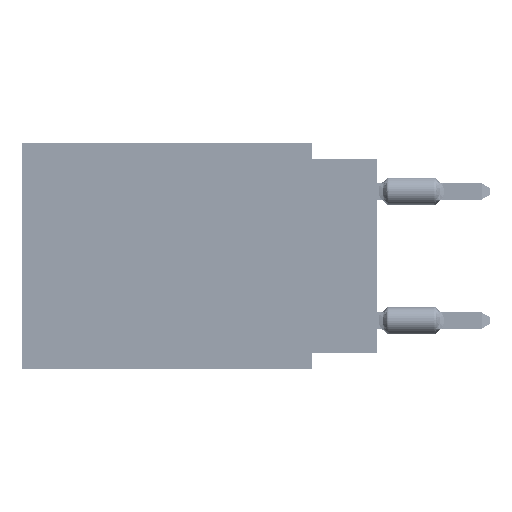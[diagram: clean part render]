
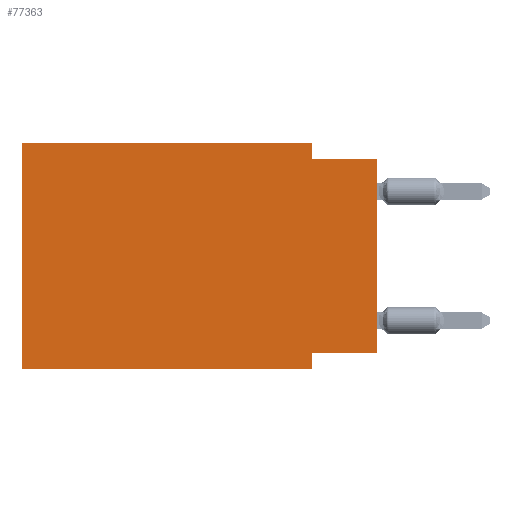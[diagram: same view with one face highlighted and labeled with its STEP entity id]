
A CAD part, left-side view. The second image highlights one B-rep face of the part: STEP entity #77363.
In plain terms, the highlighted planar face has unit normal (-1, 0, 0).
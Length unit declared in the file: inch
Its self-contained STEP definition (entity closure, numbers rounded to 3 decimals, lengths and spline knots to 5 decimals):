
#1466 = CARTESIAN_POINT ( 'NONE',  ( 0., 0., 0. ) ) ;
#2715 = VERTEX_POINT ( 'NONE', #65678 ) ;
#2759 = VECTOR ( 'NONE', #13557, 39.37008 ) ;
#5879 = CARTESIAN_POINT ( 'NONE',  ( 0., 0.1, 0. ) ) ;
#6852 = VECTOR ( 'NONE', #79138, 39.37008 ) ;
#10393 = ORIENTED_EDGE ( 'NONE', *, *, #46786, .F. ) ;
#11688 = ORIENTED_EDGE ( 'NONE', *, *, #19786, .F. ) ;
#12259 = VECTOR ( 'NONE', #74621, 39.37008 ) ;
#13557 = DIRECTION ( 'NONE',  ( 0., -1., 0. ) ) ;
#15451 = VERTEX_POINT ( 'NONE', #5879 ) ;
#16289 = LINE ( 'NONE', #46729, #67228 ) ;
#18118 = LINE ( 'NONE', #40530, #84596 ) ;
#18989 = ORIENTED_EDGE ( 'NONE', *, *, #36128, .F. ) ;
#19786 = EDGE_CURVE ( 'NONE', #51342, #15451, #20488, .T. ) ;
#20488 = LINE ( 'NONE', #79812, #2759 ) ;
#24051 = PLANE ( 'NONE',  #74735 ) ;
#24449 = VERTEX_POINT ( 'NONE', #85669 ) ;
#24643 = LINE ( 'NONE', #39053, #6852 ) ;
#25354 = FACE_OUTER_BOUND ( 'NONE', #51975, .T. ) ;
#25964 = LINE ( 'NONE', #35939, #59287 ) ;
#28844 = LINE ( 'NONE', #77173, #62168 ) ;
#29135 = VERTEX_POINT ( 'NONE', #63489 ) ;
#31354 = EDGE_CURVE ( 'NONE', #45659, #51342, #16289, .T. ) ;
#32026 = LINE ( 'NONE', #81225, #12259 ) ;
#33195 = CARTESIAN_POINT ( 'NONE',  ( 0., 0.1, -0.325 ) ) ;
#35915 = EDGE_CURVE ( 'NONE', #45659, #24449, #32026, .T. ) ;
#35939 = CARTESIAN_POINT ( 'NONE',  ( 0., 0., -0.325 ) ) ;
#36128 = EDGE_CURVE ( 'NONE', #29135, #73778, #28844, .T. ) ;
#37294 = DIRECTION ( 'NONE',  ( 0., -1., 0. ) ) ;
#37380 = DIRECTION ( 'NONE',  ( 0., 0., -1. ) ) ;
#39053 = CARTESIAN_POINT ( 'NONE',  ( 0., 0.1, 0. ) ) ;
#39264 = EDGE_CURVE ( 'NONE', #2715, #73778, #80186, .T. ) ;
#39515 = CARTESIAN_POINT ( 'NONE',  ( 0., 0.55, -0.35 ) ) ;
#40530 = CARTESIAN_POINT ( 'NONE',  ( 0., 0.1, -0.35 ) ) ;
#41360 = ORIENTED_EDGE ( 'NONE', *, *, #43000, .F. ) ;
#42317 = ORIENTED_EDGE ( 'NONE', *, *, #31354, .F. ) ;
#42715 = DIRECTION ( 'NONE',  ( 0., 1., 0. ) ) ;
#42787 = CARTESIAN_POINT ( 'NONE',  ( 0., 0.55, 0. ) ) ;
#42950 = ORIENTED_EDGE ( 'NONE', *, *, #35915, .T. ) ;
#43000 = EDGE_CURVE ( 'NONE', #59905, #24449, #18118, .T. ) ;
#45659 = VERTEX_POINT ( 'NONE', #39515 ) ;
#46729 = CARTESIAN_POINT ( 'NONE',  ( 0., 0.55, 0. ) ) ;
#46786 = EDGE_CURVE ( 'NONE', #15451, #29135, #24643, .T. ) ;
#51082 = CARTESIAN_POINT ( 'NONE',  ( 0., 0., -0.025 ) ) ;
#51342 = VERTEX_POINT ( 'NONE', #42787 ) ;
#51975 = EDGE_LOOP ( 'NONE', ( #81261, #18989, #10393, #11688, #42317, #42950, #41360, #65138 ) ) ;
#53350 = DIRECTION ( 'NONE',  ( 0., 0., 1. ) ) ;
#59287 = VECTOR ( 'NONE', #42715, 39.37008 ) ;
#59905 = VERTEX_POINT ( 'NONE', #33195 ) ;
#60601 = DIRECTION ( 'NONE',  ( 0., 0., -1. ) ) ;
#61397 = DIRECTION ( 'NONE',  ( 0., 0., 1. ) ) ;
#62168 = VECTOR ( 'NONE', #37294, 39.37008 ) ;
#62581 = VECTOR ( 'NONE', #61397, 39.37008 ) ;
#63489 = CARTESIAN_POINT ( 'NONE',  ( 0., 0.1, -0.025 ) ) ;
#65138 = ORIENTED_EDGE ( 'NONE', *, *, #72108, .F. ) ;
#65678 = CARTESIAN_POINT ( 'NONE',  ( 0., 0., -0.325 ) ) ;
#67228 = VECTOR ( 'NONE', #53350, 39.37008 ) ;
#70573 = CARTESIAN_POINT ( 'NONE',  ( 0., 0.55, 0. ) ) ;
#72108 = EDGE_CURVE ( 'NONE', #2715, #59905, #25964, .T. ) ;
#73778 = VERTEX_POINT ( 'NONE', #51082 ) ;
#74621 = DIRECTION ( 'NONE',  ( 0., -1., 0. ) ) ;
#74735 = AXIS2_PLACEMENT_3D ( 'NONE', #70573, #77258, #37380 ) ;
#77173 = CARTESIAN_POINT ( 'NONE',  ( 0., 0., -0.025 ) ) ;
#77258 = DIRECTION ( 'NONE',  ( 1., 0., 0. ) ) ;
#77363 = ADVANCED_FACE ( 'NONE', ( #25354 ), #24051, .F. ) ;
#79138 = DIRECTION ( 'NONE',  ( 0., 0., -1. ) ) ;
#79812 = CARTESIAN_POINT ( 'NONE',  ( 0., 0.55, 0. ) ) ;
#80186 = LINE ( 'NONE', #1466, #62581 ) ;
#81225 = CARTESIAN_POINT ( 'NONE',  ( 0., 0.55, -0.35 ) ) ;
#81261 = ORIENTED_EDGE ( 'NONE', *, *, #39264, .T. ) ;
#84596 = VECTOR ( 'NONE', #60601, 39.37008 ) ;
#85669 = CARTESIAN_POINT ( 'NONE',  ( 0., 0.1, -0.35 ) ) ;
